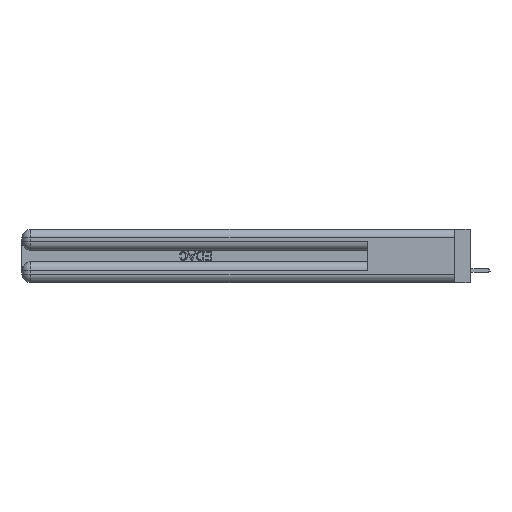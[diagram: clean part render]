
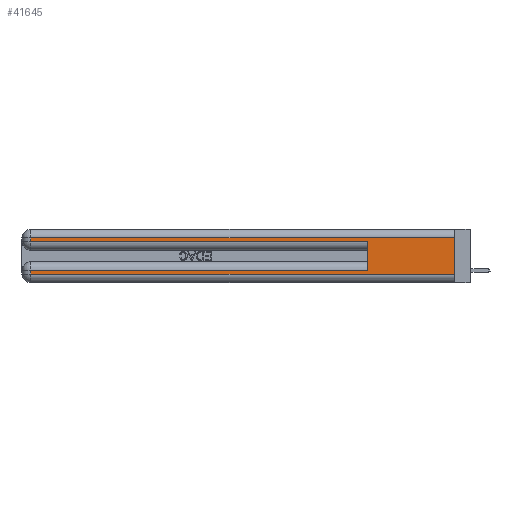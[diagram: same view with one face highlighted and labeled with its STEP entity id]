
A CAD part, left-side view. The second image highlights one B-rep face of the part: STEP entity #41645.
In plain terms, the highlighted planar face has unit normal (-1, 0, 0).
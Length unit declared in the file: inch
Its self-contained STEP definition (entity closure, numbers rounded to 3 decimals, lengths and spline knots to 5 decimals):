
#181 = CARTESIAN_POINT ( 'NONE',  ( 0., 0.6, 0.145 ) ) ;
#930 = VERTEX_POINT ( 'NONE', #41714 ) ;
#1344 = VECTOR ( 'NONE', #45866, 39.37008 ) ;
#5111 = CARTESIAN_POINT ( 'NONE',  ( 0., 0., 0.31 ) ) ;
#5366 = LINE ( 'NONE', #45700, #1344 ) ;
#5617 = DIRECTION ( 'NONE',  ( 0., 1., 0. ) ) ;
#6948 = CARTESIAN_POINT ( 'NONE',  ( 0., 2.94, 0.06 ) ) ;
#7495 = DIRECTION ( 'NONE',  ( 1., 0., 0. ) ) ;
#8907 = ORIENTED_EDGE ( 'NONE', *, *, #38547, .F. ) ;
#9084 = EDGE_CURVE ( 'NONE', #23065, #11161, #22549, .T. ) ;
#9426 = EDGE_CURVE ( 'NONE', #47752, #41681, #14436, .T. ) ;
#10184 = CARTESIAN_POINT ( 'NONE',  ( 0., 0., 0.37 ) ) ;
#10806 = CARTESIAN_POINT ( 'NONE',  ( 0., 0.6, 0.085 ) ) ;
#11161 = VERTEX_POINT ( 'NONE', #6948 ) ;
#11791 = CARTESIAN_POINT ( 'NONE',  ( 0., 0., 0.06 ) ) ;
#11803 = VECTOR ( 'NONE', #33608, 39.37008 ) ;
#13177 = CARTESIAN_POINT ( 'NONE',  ( 0., 0., 0.31 ) ) ;
#14207 = LINE ( 'NONE', #181, #11803 ) ;
#14436 = LINE ( 'NONE', #5111, #41686 ) ;
#14906 = DIRECTION ( 'NONE',  ( 0., 0., -1. ) ) ;
#15448 = EDGE_CURVE ( 'NONE', #41681, #20427, #20579, .T. ) ;
#16484 = ORIENTED_EDGE ( 'NONE', *, *, #20910, .F. ) ;
#18441 = DIRECTION ( 'NONE',  ( 0., 1., 0. ) ) ;
#19905 = ORIENTED_EDGE ( 'NONE', *, *, #15448, .T. ) ;
#20079 = VECTOR ( 'NONE', #28509, 39.37008 ) ;
#20427 = VERTEX_POINT ( 'NONE', #36271 ) ;
#20579 = LINE ( 'NONE', #29391, #47910 ) ;
#20910 = EDGE_CURVE ( 'NONE', #47752, #41617, #47434, .T. ) ;
#22524 = EDGE_LOOP ( 'NONE', ( #16484, #39019, #19905, #32153, #8907, #44218, #31537, #28182 ) ) ;
#22549 = LINE ( 'NONE', #41028, #29576 ) ;
#22670 = DIRECTION ( 'NONE',  ( 0., 0., -1. ) ) ;
#22673 = FACE_OUTER_BOUND ( 'NONE', #22524, .T. ) ;
#23065 = VERTEX_POINT ( 'NONE', #31142 ) ;
#25388 = VECTOR ( 'NONE', #18441, 39.37008 ) ;
#25796 = DIRECTION ( 'NONE',  ( 0., 0., -1. ) ) ;
#28182 = ORIENTED_EDGE ( 'NONE', *, *, #33430, .T. ) ;
#28210 = AXIS2_PLACEMENT_3D ( 'NONE', #45067, #7495, #22670 ) ;
#28509 = DIRECTION ( 'NONE',  ( 0., 0., -1. ) ) ;
#29391 = CARTESIAN_POINT ( 'NONE',  ( 0., 2.94, 0.37 ) ) ;
#29576 = VECTOR ( 'NONE', #14906, 39.37008 ) ;
#30154 = CARTESIAN_POINT ( 'NONE',  ( 0., 2.94, 0.31 ) ) ;
#31142 = CARTESIAN_POINT ( 'NONE',  ( 0., 2.94, 0.085 ) ) ;
#31537 = ORIENTED_EDGE ( 'NONE', *, *, #9084, .T. ) ;
#31559 = VECTOR ( 'NONE', #42138, 39.37008 ) ;
#32153 = ORIENTED_EDGE ( 'NONE', *, *, #40805, .T. ) ;
#33430 = EDGE_CURVE ( 'NONE', #11161, #41617, #40795, .T. ) ;
#33608 = DIRECTION ( 'NONE',  ( 0., 0., 1. ) ) ;
#36271 = CARTESIAN_POINT ( 'NONE',  ( 0., 2.94, 0.285 ) ) ;
#37453 = PLANE ( 'NONE',  #28210 ) ;
#38082 = CARTESIAN_POINT ( 'NONE',  ( 0., 0., 0.06 ) ) ;
#38547 = EDGE_CURVE ( 'NONE', #42735, #930, #14207, .T. ) ;
#39019 = ORIENTED_EDGE ( 'NONE', *, *, #9426, .T. ) ;
#40469 = LINE ( 'NONE', #48000, #25388 ) ;
#40795 = LINE ( 'NONE', #38082, #31559 ) ;
#40805 = EDGE_CURVE ( 'NONE', #20427, #930, #5366, .T. ) ;
#41028 = CARTESIAN_POINT ( 'NONE',  ( 0., 2.94, 0.37 ) ) ;
#41617 = VERTEX_POINT ( 'NONE', #11791 ) ;
#41645 = ADVANCED_FACE ( 'NONE', ( #22673 ), #37453, .F. ) ;
#41681 = VERTEX_POINT ( 'NONE', #30154 ) ;
#41686 = VECTOR ( 'NONE', #5617, 39.37008 ) ;
#41714 = CARTESIAN_POINT ( 'NONE',  ( 0., 0.6, 0.285 ) ) ;
#42138 = DIRECTION ( 'NONE',  ( 0., -1., 0. ) ) ;
#42735 = VERTEX_POINT ( 'NONE', #10806 ) ;
#44045 = EDGE_CURVE ( 'NONE', #42735, #23065, #40469, .T. ) ;
#44218 = ORIENTED_EDGE ( 'NONE', *, *, #44045, .T. ) ;
#45067 = CARTESIAN_POINT ( 'NONE',  ( 0., 0., 0.37 ) ) ;
#45700 = CARTESIAN_POINT ( 'NONE',  ( 0., 0., 0.285 ) ) ;
#45866 = DIRECTION ( 'NONE',  ( 0., -1., 0. ) ) ;
#47434 = LINE ( 'NONE', #10184, #20079 ) ;
#47752 = VERTEX_POINT ( 'NONE', #13177 ) ;
#47910 = VECTOR ( 'NONE', #25796, 39.37008 ) ;
#48000 = CARTESIAN_POINT ( 'NONE',  ( 0., 0., 0.085 ) ) ;
